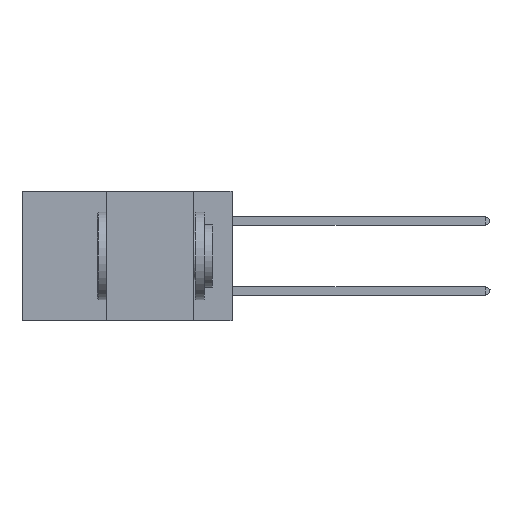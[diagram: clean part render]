
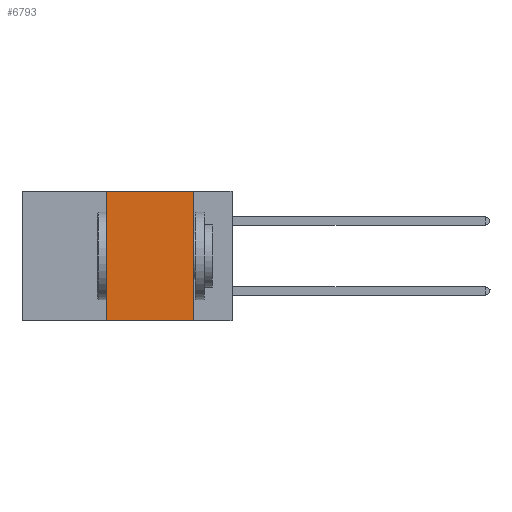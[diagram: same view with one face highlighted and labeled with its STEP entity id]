
A CAD part, left-side view. The second image highlights one B-rep face of the part: STEP entity #6793.
In plain terms, the highlighted planar face has unit normal (-1, 0, 0).
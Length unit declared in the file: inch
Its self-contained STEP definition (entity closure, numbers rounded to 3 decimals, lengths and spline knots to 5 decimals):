
#714 = EDGE_LOOP ( 'NONE', ( #11834, #7256, #737, #7271 ) ) ;
#720 = VERTEX_POINT ( 'NONE', #9067 ) ;
#737 = ORIENTED_EDGE ( 'NONE', *, *, #11851, .F. ) ;
#757 = DIRECTION ( 'NONE',  ( 0., 0., 1. ) ) ;
#1000 = LINE ( 'NONE', #4719, #9423 ) ;
#1229 = VECTOR ( 'NONE', #5176, 39.37008 ) ;
#1244 = FACE_OUTER_BOUND ( 'NONE', #714, .T. ) ;
#1875 = CARTESIAN_POINT ( 'NONE',  ( 0., 0.11, 0. ) ) ;
#2157 = VERTEX_POINT ( 'NONE', #7419 ) ;
#2511 = CARTESIAN_POINT ( 'NONE',  ( 0., 0.6, 0. ) ) ;
#3534 = EDGE_CURVE ( 'NONE', #720, #9162, #1000, .T. ) ;
#4066 = CARTESIAN_POINT ( 'NONE',  ( 0., 0.36, 0. ) ) ;
#4155 = LINE ( 'NONE', #13417, #9620 ) ;
#4692 = LINE ( 'NONE', #4066, #6789 ) ;
#4709 = DIRECTION ( 'NONE',  ( 0., -1., 0. ) ) ;
#4719 = CARTESIAN_POINT ( 'NONE',  ( 0., 0.6, 0. ) ) ;
#4836 = LINE ( 'NONE', #1875, #1229 ) ;
#5176 = DIRECTION ( 'NONE',  ( 0., 0., -1. ) ) ;
#6789 = VECTOR ( 'NONE', #757, 39.37008 ) ;
#6793 = ADVANCED_FACE ( 'NONE', ( #1244 ), #9810, .F. ) ;
#6805 = DIRECTION ( 'NONE',  ( 0., 0., -1. ) ) ;
#6884 = VERTEX_POINT ( 'NONE', #6995 ) ;
#6995 = CARTESIAN_POINT ( 'NONE',  ( 0., 0.36, -0.37 ) ) ;
#7225 = EDGE_CURVE ( 'NONE', #6884, #2157, #4155, .T. ) ;
#7256 = ORIENTED_EDGE ( 'NONE', *, *, #3534, .F. ) ;
#7271 = ORIENTED_EDGE ( 'NONE', *, *, #7225, .T. ) ;
#7419 = CARTESIAN_POINT ( 'NONE',  ( 0., 0.11, -0.37 ) ) ;
#7461 = DIRECTION ( 'NONE',  ( 0., -1., 0. ) ) ;
#7801 = AXIS2_PLACEMENT_3D ( 'NONE', #2511, #12760, #6805 ) ;
#9067 = CARTESIAN_POINT ( 'NONE',  ( 0., 0.36, 0. ) ) ;
#9162 = VERTEX_POINT ( 'NONE', #11664 ) ;
#9423 = VECTOR ( 'NONE', #4709, 39.37008 ) ;
#9620 = VECTOR ( 'NONE', #7461, 39.37008 ) ;
#9810 = PLANE ( 'NONE',  #7801 ) ;
#11664 = CARTESIAN_POINT ( 'NONE',  ( 0., 0.11, 0. ) ) ;
#11834 = ORIENTED_EDGE ( 'NONE', *, *, #13150, .F. ) ;
#11851 = EDGE_CURVE ( 'NONE', #6884, #720, #4692, .T. ) ;
#12760 = DIRECTION ( 'NONE',  ( 1., 0., 0. ) ) ;
#13150 = EDGE_CURVE ( 'NONE', #9162, #2157, #4836, .T. ) ;
#13417 = CARTESIAN_POINT ( 'NONE',  ( 0., 0.6, -0.37 ) ) ;
